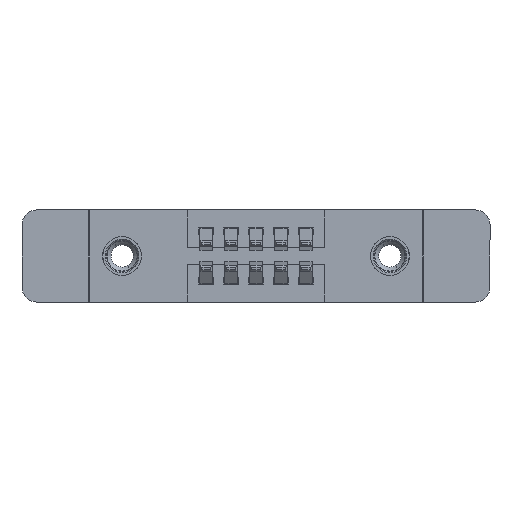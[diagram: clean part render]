
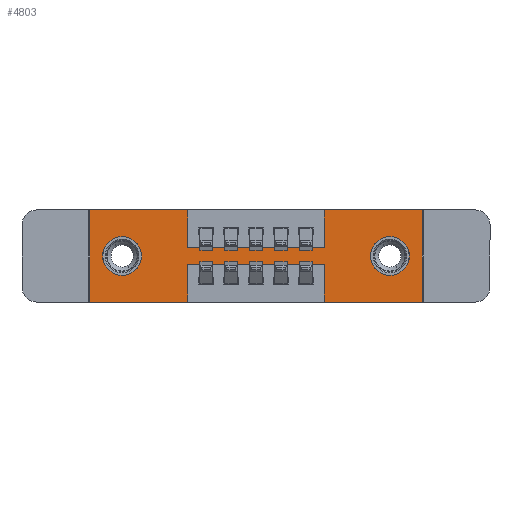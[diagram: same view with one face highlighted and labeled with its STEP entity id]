
A CAD part, front view. The second image highlights one B-rep face of the part: STEP entity #4803.
In plain terms, the highlighted planar face has unit normal (0, -1, 0).
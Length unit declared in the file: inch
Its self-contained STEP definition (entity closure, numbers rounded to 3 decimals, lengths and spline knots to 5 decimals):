
#108 = VERTEX_POINT ( 'NONE', #11882 ) ;
#166 = ORIENTED_EDGE ( 'NONE', *, *, #9860, .T. ) ;
#557 = VERTEX_POINT ( 'NONE', #9031 ) ;
#622 = CARTESIAN_POINT ( 'NONE',  ( 1.205, 0., -0.263 ) ) ;
#636 = CARTESIAN_POINT ( 'NONE',  ( 1.205, 0., -0.185 ) ) ;
#706 = ORIENTED_EDGE ( 'NONE', *, *, #13823, .F. ) ;
#839 = ORIENTED_EDGE ( 'NONE', *, *, #6870, .F. ) ;
#885 = VERTEX_POINT ( 'NONE', #6967 ) ;
#1021 = VERTEX_POINT ( 'NONE', #6023 ) ;
#1090 = VECTOR ( 'NONE', #5637, 39.37008 ) ;
#1170 = CARTESIAN_POINT ( 'NONE',  ( 0.9425, 0., -0.37 ) ) ;
#1195 = ORIENTED_EDGE ( 'NONE', *, *, #4043, .F. ) ;
#1260 = VERTEX_POINT ( 'NONE', #4038 ) ;
#1279 = AXIS2_PLACEMENT_3D ( 'NONE', #2883, #6293, #13684 ) ;
#1281 = CARTESIAN_POINT ( 'NONE',  ( 0.13, 0., -0.185 ) ) ;
#1295 = ORIENTED_EDGE ( 'NONE', *, *, #11902, .F. ) ;
#1434 = VECTOR ( 'NONE', #6129, 39.37008 ) ;
#1838 = DIRECTION ( 'NONE',  ( 0., 0., -1. ) ) ;
#2469 = CARTESIAN_POINT ( 'NONE',  ( 0.3925, 0., -0.37 ) ) ;
#2473 = DIRECTION ( 'NONE',  ( 0., 0., 1. ) ) ;
#2794 = EDGE_CURVE ( 'NONE', #557, #11027, #13886, .T. ) ;
#2797 = VECTOR ( 'NONE', #6566, 39.37008 ) ;
#2883 = CARTESIAN_POINT ( 'NONE',  ( 0., 0., -0.37 ) ) ;
#2979 = CARTESIAN_POINT ( 'NONE',  ( 0.3925, 0., -0.22 ) ) ;
#3051 = LINE ( 'NONE', #6885, #8637 ) ;
#3161 = DIRECTION ( 'NONE',  ( 1., 0., 0. ) ) ;
#3216 = VERTEX_POINT ( 'NONE', #3714 ) ;
#3365 = CARTESIAN_POINT ( 'NONE',  ( 0.3925, 0., -0.37 ) ) ;
#3571 = VERTEX_POINT ( 'NONE', #2469 ) ;
#3688 = CARTESIAN_POINT ( 'NONE',  ( 0.3925, 0., 0. ) ) ;
#3714 = CARTESIAN_POINT ( 'NONE',  ( 0.13, 0., -0.107 ) ) ;
#3762 = EDGE_CURVE ( 'NONE', #885, #3820, #14167, .T. ) ;
#3800 = VERTEX_POINT ( 'NONE', #12612 ) ;
#3820 = VERTEX_POINT ( 'NONE', #12655 ) ;
#3947 = CARTESIAN_POINT ( 'NONE',  ( 0., 0., 0. ) ) ;
#4038 = CARTESIAN_POINT ( 'NONE',  ( 0.3925, 0., -0.15 ) ) ;
#4043 = EDGE_CURVE ( 'NONE', #3800, #1260, #13696, .T. ) ;
#4107 = DIRECTION ( 'NONE',  ( 0., 0., -1. ) ) ;
#4114 = VERTEX_POINT ( 'NONE', #4967 ) ;
#4122 = CIRCLE ( 'NONE', #6095, 0.078 ) ;
#4163 = EDGE_CURVE ( 'NONE', #4114, #8053, #10322, .T. ) ;
#4303 = ORIENTED_EDGE ( 'NONE', *, *, #12372, .F. ) ;
#4382 = CARTESIAN_POINT ( 'NONE',  ( 0., 0., -0.37 ) ) ;
#4390 = CARTESIAN_POINT ( 'NONE',  ( 0.13, 0., -0.185 ) ) ;
#4535 = ORIENTED_EDGE ( 'NONE', *, *, #4956, .T. ) ;
#4803 = ADVANCED_FACE ( 'NONE', ( #11955, #6956, #9488 ), #5195, .T. ) ;
#4956 = EDGE_CURVE ( 'NONE', #1021, #3216, #10658, .T. ) ;
#4967 = CARTESIAN_POINT ( 'NONE',  ( 1.335, 0., -0.37 ) ) ;
#5128 = DIRECTION ( 'NONE',  ( 0., 0., 1. ) ) ;
#5195 = PLANE ( 'NONE',  #1279 ) ;
#5299 = CARTESIAN_POINT ( 'NONE',  ( 0.3925, 0., -0.22 ) ) ;
#5463 = CARTESIAN_POINT ( 'NONE',  ( 0.9425, 0., 0. ) ) ;
#5510 = ORIENTED_EDGE ( 'NONE', *, *, #10189, .F. ) ;
#5516 = DIRECTION ( 'NONE',  ( 0., 0., 1. ) ) ;
#5560 = VECTOR ( 'NONE', #11946, 39.37008 ) ;
#5565 = EDGE_CURVE ( 'NONE', #12527, #13176, #4122, .T. ) ;
#5637 = DIRECTION ( 'NONE',  ( 0., 0., 1. ) ) ;
#5652 = DIRECTION ( 'NONE',  ( 0., 0., -1. ) ) ;
#5820 = LINE ( 'NONE', #5463, #2797 ) ;
#5903 = AXIS2_PLACEMENT_3D ( 'NONE', #4390, #11953, #5516 ) ;
#5931 = VECTOR ( 'NONE', #3161, 39.37008 ) ;
#6023 = CARTESIAN_POINT ( 'NONE',  ( 0.13, 0., -0.263 ) ) ;
#6095 = AXIS2_PLACEMENT_3D ( 'NONE', #12719, #6350, #13740 ) ;
#6129 = DIRECTION ( 'NONE',  ( -1., 0., 0. ) ) ;
#6176 = EDGE_CURVE ( 'NONE', #3571, #885, #8829, .T. ) ;
#6282 = LINE ( 'NONE', #3365, #8858 ) ;
#6293 = DIRECTION ( 'NONE',  ( 0., -1., 0. ) ) ;
#6347 = EDGE_CURVE ( 'NONE', #3820, #3800, #9643, .T. ) ;
#6350 = DIRECTION ( 'NONE',  ( 0., 1., 0. ) ) ;
#6566 = DIRECTION ( 'NONE',  ( 0., 0., 1. ) ) ;
#6601 = ORIENTED_EDGE ( 'NONE', *, *, #12716, .T. ) ;
#6870 = EDGE_CURVE ( 'NONE', #1260, #11779, #3051, .T. ) ;
#6885 = CARTESIAN_POINT ( 'NONE',  ( 0.3925, 0., -0.15 ) ) ;
#6956 = FACE_BOUND ( 'NONE', #13988, .T. ) ;
#6967 = CARTESIAN_POINT ( 'NONE',  ( 0., 0., -0.37 ) ) ;
#7209 = VECTOR ( 'NONE', #4107, 39.37008 ) ;
#7627 = EDGE_LOOP ( 'NONE', ( #10975, #6601 ) ) ;
#7647 = CARTESIAN_POINT ( 'NONE',  ( 0.9425, 0., -0.15 ) ) ;
#7965 = CARTESIAN_POINT ( 'NONE',  ( 0., 0., 0. ) ) ;
#8053 = VERTEX_POINT ( 'NONE', #1170 ) ;
#8488 = DIRECTION ( 'NONE',  ( -1., 0., 0. ) ) ;
#8563 = DIRECTION ( 'NONE',  ( 0., 1., 0. ) ) ;
#8637 = VECTOR ( 'NONE', #9071, 39.37008 ) ;
#8783 = ORIENTED_EDGE ( 'NONE', *, *, #10298, .F. ) ;
#8829 = LINE ( 'NONE', #4382, #5560 ) ;
#8858 = VECTOR ( 'NONE', #5652, 39.37008 ) ;
#9005 = VECTOR ( 'NONE', #5128, 39.37008 ) ;
#9031 = CARTESIAN_POINT ( 'NONE',  ( 0.9425, 0., -0.22 ) ) ;
#9071 = DIRECTION ( 'NONE',  ( 1., 0., 0. ) ) ;
#9143 = DIRECTION ( 'NONE',  ( 0., 1., 0. ) ) ;
#9488 = FACE_OUTER_BOUND ( 'NONE', #10809, .T. ) ;
#9643 = LINE ( 'NONE', #7965, #12106 ) ;
#9860 = EDGE_CURVE ( 'NONE', #3216, #1021, #11231, .T. ) ;
#10189 = EDGE_CURVE ( 'NONE', #108, #4114, #13456, .T. ) ;
#10298 = EDGE_CURVE ( 'NONE', #11779, #11206, #5820, .T. ) ;
#10322 = LINE ( 'NONE', #12519, #1434 ) ;
#10658 = CIRCLE ( 'NONE', #5903, 0.078 ) ;
#10738 = ORIENTED_EDGE ( 'NONE', *, *, #2794, .F. ) ;
#10809 = EDGE_LOOP ( 'NONE', ( #1295, #10738, #706, #13772, #5510, #4303, #8783, #839, #1195, #12733, #13695, #11657 ) ) ;
#10975 = ORIENTED_EDGE ( 'NONE', *, *, #5565, .T. ) ;
#10981 = VECTOR ( 'NONE', #13401, 39.37008 ) ;
#11027 = VERTEX_POINT ( 'NONE', #5299 ) ;
#11206 = VERTEX_POINT ( 'NONE', #13079 ) ;
#11231 = CIRCLE ( 'NONE', #11528, 0.078 ) ;
#11528 = AXIS2_PLACEMENT_3D ( 'NONE', #1281, #9143, #2473 ) ;
#11645 = LINE ( 'NONE', #13884, #5931 ) ;
#11657 = ORIENTED_EDGE ( 'NONE', *, *, #6176, .F. ) ;
#11719 = CARTESIAN_POINT ( 'NONE',  ( 1.335, 0., 0. ) ) ;
#11779 = VERTEX_POINT ( 'NONE', #7647 ) ;
#11882 = CARTESIAN_POINT ( 'NONE',  ( 1.335, 0., 0. ) ) ;
#11902 = EDGE_CURVE ( 'NONE', #11027, #3571, #6282, .T. ) ;
#11946 = DIRECTION ( 'NONE',  ( -1., 0., 0. ) ) ;
#11953 = DIRECTION ( 'NONE',  ( 0., 1., 0. ) ) ;
#11955 = FACE_BOUND ( 'NONE', #7627, .T. ) ;
#12106 = VECTOR ( 'NONE', #14188, 39.37008 ) ;
#12113 = CARTESIAN_POINT ( 'NONE',  ( 0.9425, 0., -0.37 ) ) ;
#12372 = EDGE_CURVE ( 'NONE', #11206, #108, #11645, .T. ) ;
#12471 = LINE ( 'NONE', #12113, #1090 ) ;
#12519 = CARTESIAN_POINT ( 'NONE',  ( 0., 0., -0.37 ) ) ;
#12527 = VERTEX_POINT ( 'NONE', #13169 ) ;
#12612 = CARTESIAN_POINT ( 'NONE',  ( 0.3925, 0., 0. ) ) ;
#12655 = CARTESIAN_POINT ( 'NONE',  ( 0., 0., 0. ) ) ;
#12716 = EDGE_CURVE ( 'NONE', #13176, #12527, #14060, .T. ) ;
#12719 = CARTESIAN_POINT ( 'NONE',  ( 1.205, 0., -0.185 ) ) ;
#12733 = ORIENTED_EDGE ( 'NONE', *, *, #6347, .F. ) ;
#13079 = CARTESIAN_POINT ( 'NONE',  ( 0.9425, 0., 0. ) ) ;
#13169 = CARTESIAN_POINT ( 'NONE',  ( 1.205, 0., -0.107 ) ) ;
#13176 = VERTEX_POINT ( 'NONE', #622 ) ;
#13338 = AXIS2_PLACEMENT_3D ( 'NONE', #636, #8563, #1838 ) ;
#13401 = DIRECTION ( 'NONE',  ( 0., 0., -1. ) ) ;
#13456 = LINE ( 'NONE', #11719, #7209 ) ;
#13567 = VECTOR ( 'NONE', #8488, 39.37008 ) ;
#13684 = DIRECTION ( 'NONE',  ( 0., 0., -1. ) ) ;
#13695 = ORIENTED_EDGE ( 'NONE', *, *, #3762, .F. ) ;
#13696 = LINE ( 'NONE', #3688, #10981 ) ;
#13740 = DIRECTION ( 'NONE',  ( 0., 0., -1. ) ) ;
#13772 = ORIENTED_EDGE ( 'NONE', *, *, #4163, .F. ) ;
#13823 = EDGE_CURVE ( 'NONE', #8053, #557, #12471, .T. ) ;
#13884 = CARTESIAN_POINT ( 'NONE',  ( 0., 0., 0. ) ) ;
#13886 = LINE ( 'NONE', #2979, #13567 ) ;
#13988 = EDGE_LOOP ( 'NONE', ( #166, #4535 ) ) ;
#14060 = CIRCLE ( 'NONE', #13338, 0.078 ) ;
#14167 = LINE ( 'NONE', #3947, #9005 ) ;
#14188 = DIRECTION ( 'NONE',  ( 1., 0., 0. ) ) ;
